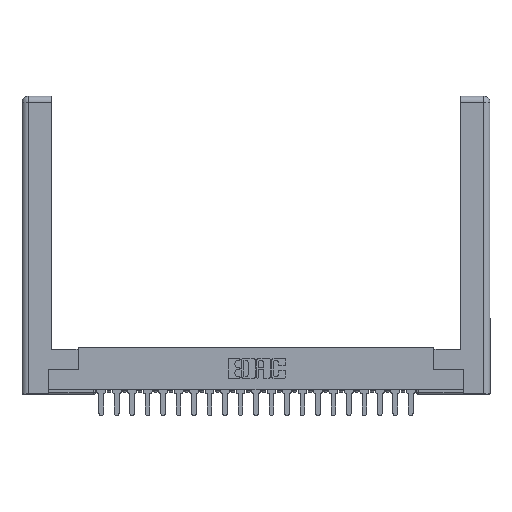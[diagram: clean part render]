
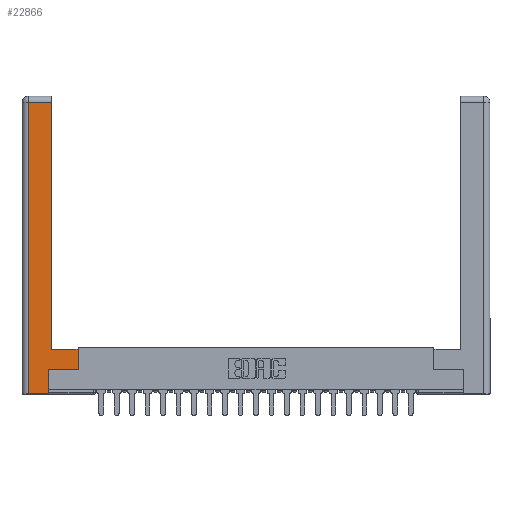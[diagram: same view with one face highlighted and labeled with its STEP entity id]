
A CAD part, top view. The second image highlights one B-rep face of the part: STEP entity #22866.
In plain terms, the highlighted planar face has unit normal (0, 0, 1).
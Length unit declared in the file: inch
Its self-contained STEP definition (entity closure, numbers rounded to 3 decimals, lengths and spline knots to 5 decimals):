
#118 = LINE ( 'NONE', #16578, #5473 ) ;
#386 = LINE ( 'NONE', #9596, #16769 ) ;
#549 = AXIS2_PLACEMENT_3D ( 'NONE', #18685, #20031, #1835 ) ;
#589 = VECTOR ( 'NONE', #18885, 39.37008 ) ;
#1129 = CARTESIAN_POINT ( 'NONE',  ( 0.565, 0.45, 0. ) ) ;
#1294 = CARTESIAN_POINT ( 'NONE',  ( 0.295, 0.45, 0. ) ) ;
#1497 = VECTOR ( 'NONE', #10961, 39.37008 ) ;
#1835 = DIRECTION ( 'NONE',  ( -1., 0., 0. ) ) ;
#1856 = CARTESIAN_POINT ( 'NONE',  ( 0.565, 0.245, 0. ) ) ;
#1898 = ORIENTED_EDGE ( 'NONE', *, *, #11574, .T. ) ;
#1931 = ORIENTED_EDGE ( 'NONE', *, *, #10209, .T. ) ;
#2039 = DIRECTION ( 'NONE',  ( 1., 0., 0. ) ) ;
#2859 = DIRECTION ( 'NONE',  ( -1., 0., 0. ) ) ;
#4679 = EDGE_CURVE ( 'NONE', #23587, #14347, #11145, .T. ) ;
#4689 = LINE ( 'NONE', #6499, #20704 ) ;
#5235 = VECTOR ( 'NONE', #19569, 39.37008 ) ;
#5417 = EDGE_CURVE ( 'NONE', #20098, #19323, #10353, .T. ) ;
#5473 = VECTOR ( 'NONE', #2039, 39.37008 ) ;
#6028 = VECTOR ( 'NONE', #14397, 39.37008 ) ;
#6499 = CARTESIAN_POINT ( 'NONE',  ( 0.0615, 2.94, 0. ) ) ;
#7339 = CARTESIAN_POINT ( 'NONE',  ( 0.565, 0.45, 0. ) ) ;
#7640 = FACE_OUTER_BOUND ( 'NONE', #9496, .T. ) ;
#7646 = DIRECTION ( 'NONE',  ( 0., 1., 0. ) ) ;
#7734 = CARTESIAN_POINT ( 'NONE',  ( 0.265, 0., 0. ) ) ;
#7849 = CARTESIAN_POINT ( 'NONE',  ( 0.295, 2.94, 0. ) ) ;
#9411 = ORIENTED_EDGE ( 'NONE', *, *, #4679, .T. ) ;
#9454 = EDGE_CURVE ( 'NONE', #9875, #19023, #17611, .T. ) ;
#9496 = EDGE_LOOP ( 'NONE', ( #19498, #22395, #9411, #17128, #1898, #22853, #23718, #1931 ) ) ;
#9596 = CARTESIAN_POINT ( 'NONE',  ( 0.265, 0., 0. ) ) ;
#9875 = VERTEX_POINT ( 'NONE', #10210 ) ;
#10209 = EDGE_CURVE ( 'NONE', #19323, #9875, #16322, .T. ) ;
#10210 = CARTESIAN_POINT ( 'NONE',  ( 0.295, 0.45, 0. ) ) ;
#10353 = LINE ( 'NONE', #1129, #1497 ) ;
#10774 = EDGE_CURVE ( 'NONE', #19023, #23587, #4689, .T. ) ;
#10781 = VERTEX_POINT ( 'NONE', #17492 ) ;
#10961 = DIRECTION ( 'NONE',  ( 0., 1., 0. ) ) ;
#11145 = LINE ( 'NONE', #11504, #589 ) ;
#11504 = CARTESIAN_POINT ( 'NONE',  ( 0.0615, 0., 0. ) ) ;
#11574 = EDGE_CURVE ( 'NONE', #12246, #10781, #15066, .T. ) ;
#12246 = VERTEX_POINT ( 'NONE', #7734 ) ;
#14347 = VERTEX_POINT ( 'NONE', #16305 ) ;
#14397 = DIRECTION ( 'NONE',  ( -1., 0., 0. ) ) ;
#14940 = PLANE ( 'NONE',  #549 ) ;
#15066 = LINE ( 'NONE', #16495, #17997 ) ;
#16305 = CARTESIAN_POINT ( 'NONE',  ( 0.0615, 0., 0. ) ) ;
#16322 = LINE ( 'NONE', #1294, #6028 ) ;
#16495 = CARTESIAN_POINT ( 'NONE',  ( 0.265, 0.245, 0. ) ) ;
#16578 = CARTESIAN_POINT ( 'NONE',  ( 0.565, 0.245, 0. ) ) ;
#16769 = VECTOR ( 'NONE', #16960, 39.37008 ) ;
#16960 = DIRECTION ( 'NONE',  ( 1., 0., 0. ) ) ;
#17128 = ORIENTED_EDGE ( 'NONE', *, *, #21714, .T. ) ;
#17492 = CARTESIAN_POINT ( 'NONE',  ( 0.265, 0.245, 0. ) ) ;
#17611 = LINE ( 'NONE', #23157, #5235 ) ;
#17997 = VECTOR ( 'NONE', #7646, 39.37008 ) ;
#18685 = CARTESIAN_POINT ( 'NONE',  ( 0., 0., 0. ) ) ;
#18814 = EDGE_CURVE ( 'NONE', #10781, #20098, #118, .T. ) ;
#18885 = DIRECTION ( 'NONE',  ( 0., -1., 0. ) ) ;
#19023 = VERTEX_POINT ( 'NONE', #7849 ) ;
#19323 = VERTEX_POINT ( 'NONE', #7339 ) ;
#19498 = ORIENTED_EDGE ( 'NONE', *, *, #9454, .T. ) ;
#19569 = DIRECTION ( 'NONE',  ( 0., 1., 0. ) ) ;
#20031 = DIRECTION ( 'NONE',  ( 0., 0., -1. ) ) ;
#20098 = VERTEX_POINT ( 'NONE', #1856 ) ;
#20704 = VECTOR ( 'NONE', #2859, 39.37008 ) ;
#21714 = EDGE_CURVE ( 'NONE', #14347, #12246, #386, .T. ) ;
#22395 = ORIENTED_EDGE ( 'NONE', *, *, #10774, .T. ) ;
#22853 = ORIENTED_EDGE ( 'NONE', *, *, #18814, .T. ) ;
#22866 = ADVANCED_FACE ( 'NONE', ( #7640 ), #14940, .F. ) ;
#23157 = CARTESIAN_POINT ( 'NONE',  ( 0.295, 3., 0. ) ) ;
#23311 = CARTESIAN_POINT ( 'NONE',  ( 0.0615, 2.94, 0. ) ) ;
#23587 = VERTEX_POINT ( 'NONE', #23311 ) ;
#23718 = ORIENTED_EDGE ( 'NONE', *, *, #5417, .T. ) ;
